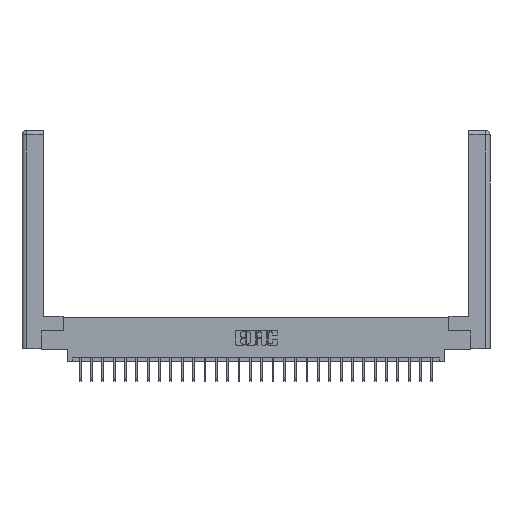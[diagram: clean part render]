
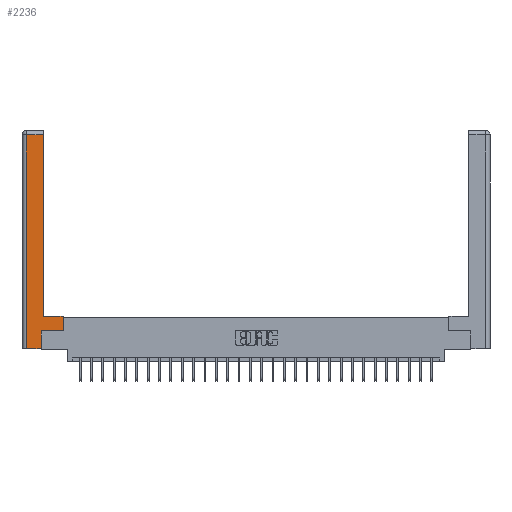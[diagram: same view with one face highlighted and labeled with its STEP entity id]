
A CAD part, top view. The second image highlights one B-rep face of the part: STEP entity #2236.
In plain terms, the highlighted planar face has unit normal (0, 0, 1).
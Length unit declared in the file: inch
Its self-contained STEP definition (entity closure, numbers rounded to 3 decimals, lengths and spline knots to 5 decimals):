
#364 = LINE ( 'NONE', #30294, #729 ) ;
#694 = CARTESIAN_POINT ( 'NONE',  ( 0.295, 0.45, 0. ) ) ;
#729 = VECTOR ( 'NONE', #11509, 39.37008 ) ;
#1383 = EDGE_LOOP ( 'NONE', ( #21023, #14019, #15721, #25312, #21594, #1519, #6306, #27235 ) ) ;
#1519 = ORIENTED_EDGE ( 'NONE', *, *, #2894, .T. ) ;
#1563 = LINE ( 'NONE', #12675, #22275 ) ;
#1770 = EDGE_CURVE ( 'NONE', #25223, #9155, #25629, .T. ) ;
#2236 = ADVANCED_FACE ( 'NONE', ( #4079 ), #25004, .F. ) ;
#2894 = EDGE_CURVE ( 'NONE', #4967, #23810, #364, .T. ) ;
#3039 = LINE ( 'NONE', #5834, #29683 ) ;
#3222 = LINE ( 'NONE', #6678, #4284 ) ;
#4079 = FACE_OUTER_BOUND ( 'NONE', #1383, .T. ) ;
#4284 = VECTOR ( 'NONE', #23217, 39.37008 ) ;
#4409 = DIRECTION ( 'NONE',  ( -1., 0., 0. ) ) ;
#4640 = EDGE_CURVE ( 'NONE', #23810, #30646, #30023, .T. ) ;
#4967 = VERTEX_POINT ( 'NONE', #18126 ) ;
#5270 = CARTESIAN_POINT ( 'NONE',  ( 0.265, 0., 0. ) ) ;
#5834 = CARTESIAN_POINT ( 'NONE',  ( 0.0615, 2.94, 0. ) ) ;
#6306 = ORIENTED_EDGE ( 'NONE', *, *, #4640, .T. ) ;
#6678 = CARTESIAN_POINT ( 'NONE',  ( 0.0615, 0., 0. ) ) ;
#6784 = CARTESIAN_POINT ( 'NONE',  ( 0.295, 0.45, 0. ) ) ;
#7779 = CARTESIAN_POINT ( 'NONE',  ( 0.265, 0.245, 0. ) ) ;
#9155 = VERTEX_POINT ( 'NONE', #18257 ) ;
#10047 = VECTOR ( 'NONE', #21481, 39.37008 ) ;
#11509 = DIRECTION ( 'NONE',  ( 1., 0., 0. ) ) ;
#12675 = CARTESIAN_POINT ( 'NONE',  ( 0.265, 0., 0. ) ) ;
#12804 = CARTESIAN_POINT ( 'NONE',  ( 0.565, 0.245, 0. ) ) ;
#14019 = ORIENTED_EDGE ( 'NONE', *, *, #25391, .T. ) ;
#14145 = VERTEX_POINT ( 'NONE', #14435 ) ;
#14359 = CARTESIAN_POINT ( 'NONE',  ( 0.295, 3., 0. ) ) ;
#14435 = CARTESIAN_POINT ( 'NONE',  ( 0.0615, 0., 0. ) ) ;
#14515 = LINE ( 'NONE', #6784, #21921 ) ;
#14605 = CARTESIAN_POINT ( 'NONE',  ( 0.565, 0.45, 0. ) ) ;
#15544 = DIRECTION ( 'NONE',  ( -1., 0., 0. ) ) ;
#15721 = ORIENTED_EDGE ( 'NONE', *, *, #29346, .T. ) ;
#17544 = DIRECTION ( 'NONE',  ( 0., 1., 0. ) ) ;
#18126 = CARTESIAN_POINT ( 'NONE',  ( 0.265, 0.245, 0. ) ) ;
#18157 = LINE ( 'NONE', #7779, #29313 ) ;
#18257 = CARTESIAN_POINT ( 'NONE',  ( 0.295, 2.94, 0. ) ) ;
#18638 = CARTESIAN_POINT ( 'NONE',  ( 0.565, 0.45, 0. ) ) ;
#20063 = EDGE_CURVE ( 'NONE', #23800, #4967, #18157, .T. ) ;
#20718 = DIRECTION ( 'NONE',  ( -1., 0., 0. ) ) ;
#20868 = CARTESIAN_POINT ( 'NONE',  ( 0.0615, 2.94, 0. ) ) ;
#21023 = ORIENTED_EDGE ( 'NONE', *, *, #1770, .T. ) ;
#21481 = DIRECTION ( 'NONE',  ( 0., 1., 0. ) ) ;
#21594 = ORIENTED_EDGE ( 'NONE', *, *, #20063, .T. ) ;
#21921 = VECTOR ( 'NONE', #4409, 39.37008 ) ;
#22275 = VECTOR ( 'NONE', #29228, 39.37008 ) ;
#23217 = DIRECTION ( 'NONE',  ( 0., -1., 0. ) ) ;
#23714 = VECTOR ( 'NONE', #23738, 39.37008 ) ;
#23738 = DIRECTION ( 'NONE',  ( 0., 1., 0. ) ) ;
#23800 = VERTEX_POINT ( 'NONE', #5270 ) ;
#23810 = VERTEX_POINT ( 'NONE', #12804 ) ;
#24673 = VERTEX_POINT ( 'NONE', #20868 ) ;
#25004 = PLANE ( 'NONE',  #28976 ) ;
#25120 = EDGE_CURVE ( 'NONE', #30646, #25223, #14515, .T. ) ;
#25213 = EDGE_CURVE ( 'NONE', #14145, #23800, #1563, .T. ) ;
#25223 = VERTEX_POINT ( 'NONE', #694 ) ;
#25312 = ORIENTED_EDGE ( 'NONE', *, *, #25213, .T. ) ;
#25391 = EDGE_CURVE ( 'NONE', #9155, #24673, #3039, .T. ) ;
#25629 = LINE ( 'NONE', #14359, #10047 ) ;
#27227 = CARTESIAN_POINT ( 'NONE',  ( 0., 0., 0. ) ) ;
#27235 = ORIENTED_EDGE ( 'NONE', *, *, #25120, .T. ) ;
#28976 = AXIS2_PLACEMENT_3D ( 'NONE', #27227, #30383, #20718 ) ;
#29228 = DIRECTION ( 'NONE',  ( 1., 0., 0. ) ) ;
#29313 = VECTOR ( 'NONE', #17544, 39.37008 ) ;
#29346 = EDGE_CURVE ( 'NONE', #24673, #14145, #3222, .T. ) ;
#29683 = VECTOR ( 'NONE', #15544, 39.37008 ) ;
#30023 = LINE ( 'NONE', #18638, #23714 ) ;
#30294 = CARTESIAN_POINT ( 'NONE',  ( 0.565, 0.245, 0. ) ) ;
#30383 = DIRECTION ( 'NONE',  ( 0., 0., -1. ) ) ;
#30646 = VERTEX_POINT ( 'NONE', #14605 ) ;
